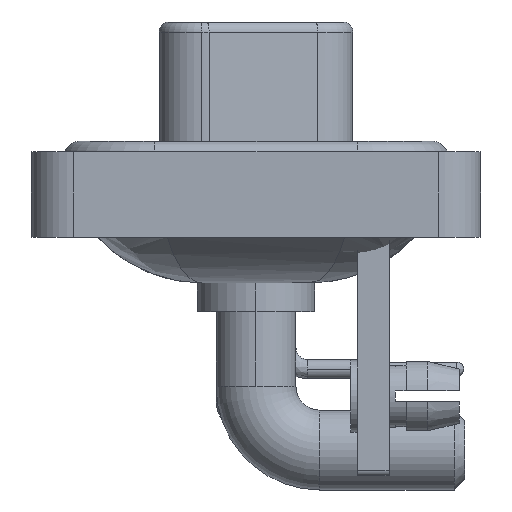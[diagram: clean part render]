
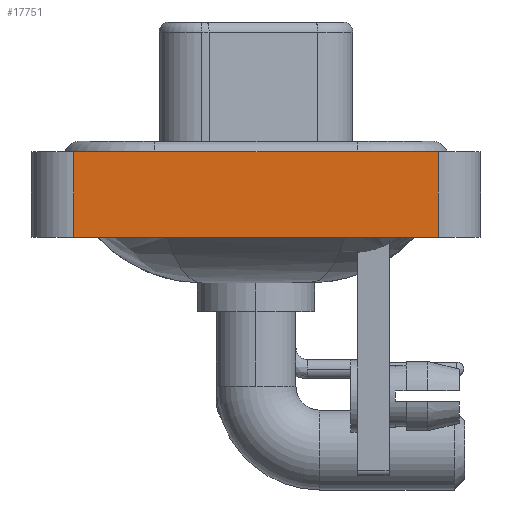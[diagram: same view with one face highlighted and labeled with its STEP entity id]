
A CAD part, left-side view. The second image highlights one B-rep face of the part: STEP entity #17751.
In plain terms, the highlighted planar face has unit normal (-1, 0, 0).
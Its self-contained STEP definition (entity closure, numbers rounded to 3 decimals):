
#17 = VERTEX_POINT ( 'NONE', #9977 ) ;
#895 = ORIENTED_EDGE ( 'NONE', *, *, #8391, .F. ) ;
#1260 = CARTESIAN_POINT ( 'NONE',  ( -7.35, -8.55, -3.6 ) ) ;
#1664 = DIRECTION ( 'NONE',  ( -1., 0., 0. ) ) ;
#1688 = AXIS2_PLACEMENT_3D ( 'NONE', #28469, #1664, #7138 ) ;
#2067 = CARTESIAN_POINT ( 'NONE',  ( -7.35, 8.55, -3.6 ) ) ;
#4792 = PLANE ( 'NONE',  #1688 ) ;
#5513 = ORIENTED_EDGE ( 'NONE', *, *, #9881, .T. ) ;
#5661 = DIRECTION ( 'NONE',  ( 0., -1., 0. ) ) ;
#6423 = VECTOR ( 'NONE', #27764, 1000. ) ;
#6785 = DIRECTION ( 'NONE',  ( 0., 0., 1. ) ) ;
#7077 = VERTEX_POINT ( 'NONE', #24761 ) ;
#7138 = DIRECTION ( 'NONE',  ( 0., 0., 1. ) ) ;
#7666 = EDGE_LOOP ( 'NONE', ( #19888, #30089, #895, #5513 ) ) ;
#8391 = EDGE_CURVE ( 'NONE', #7077, #17245, #16227, .T. ) ;
#9881 = EDGE_CURVE ( 'NONE', #7077, #17, #11641, .T. ) ;
#9977 = CARTESIAN_POINT ( 'NONE',  ( -7.35, -8.55, -3.6 ) ) ;
#10651 = VERTEX_POINT ( 'NONE', #24045 ) ;
#11641 = LINE ( 'NONE', #12472, #28951 ) ;
#12077 = EDGE_CURVE ( 'NONE', #17245, #10651, #23923, .T. ) ;
#12472 = CARTESIAN_POINT ( 'NONE',  ( -7.35, -8.55, -3.6 ) ) ;
#13795 = FACE_OUTER_BOUND ( 'NONE', #7666, .T. ) ;
#14516 = CARTESIAN_POINT ( 'NONE',  ( -7.35, -8.55, 0.4 ) ) ;
#15376 = EDGE_CURVE ( 'NONE', #17, #10651, #20397, .T. ) ;
#16227 = LINE ( 'NONE', #2067, #26353 ) ;
#17245 = VERTEX_POINT ( 'NONE', #22576 ) ;
#17751 = ADVANCED_FACE ( 'NONE', ( #13795 ), #4792, .T. ) ;
#19888 = ORIENTED_EDGE ( 'NONE', *, *, #15376, .T. ) ;
#20397 = LINE ( 'NONE', #1260, #6423 ) ;
#21105 = DIRECTION ( 'NONE',  ( 0., -1., 0. ) ) ;
#22576 = CARTESIAN_POINT ( 'NONE',  ( -7.35, 8.55, 0.4 ) ) ;
#22720 = VECTOR ( 'NONE', #5661, 1000. ) ;
#23923 = LINE ( 'NONE', #14516, #22720 ) ;
#24045 = CARTESIAN_POINT ( 'NONE',  ( -7.35, -8.55, 0.4 ) ) ;
#24761 = CARTESIAN_POINT ( 'NONE',  ( -7.35, 8.55, -3.6 ) ) ;
#26353 = VECTOR ( 'NONE', #6785, 1000. ) ;
#27764 = DIRECTION ( 'NONE',  ( 0., 0., 1. ) ) ;
#28469 = CARTESIAN_POINT ( 'NONE',  ( -7.35, -8.55, -3.6 ) ) ;
#28951 = VECTOR ( 'NONE', #21105, 1000. ) ;
#30089 = ORIENTED_EDGE ( 'NONE', *, *, #12077, .F. ) ;
